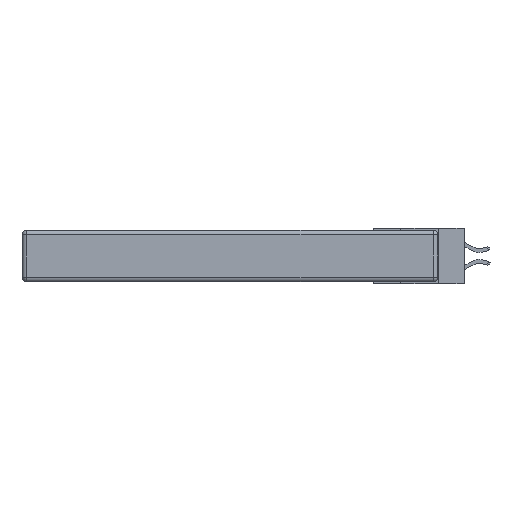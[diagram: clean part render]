
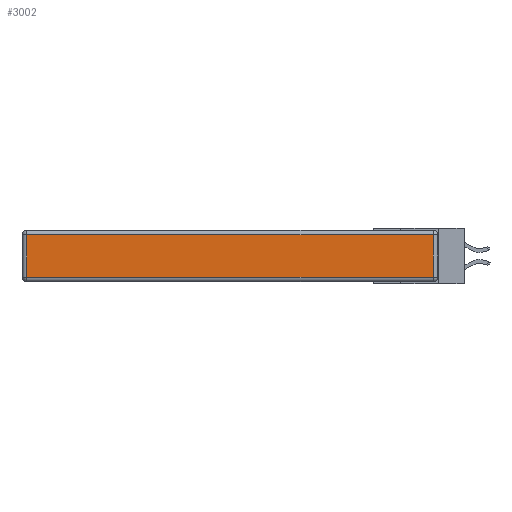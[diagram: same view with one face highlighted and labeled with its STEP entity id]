
A CAD part, left-side view. The second image highlights one B-rep face of the part: STEP entity #3002.
In plain terms, the highlighted planar face has unit normal (-1, 0, 0).
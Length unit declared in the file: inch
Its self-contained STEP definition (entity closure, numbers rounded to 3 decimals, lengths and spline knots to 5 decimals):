
#45 = AXIS2_PLACEMENT_3D ( 'NONE', #1688, #13537, #12020 ) ;
#540 = LINE ( 'NONE', #4034, #991 ) ;
#648 = CARTESIAN_POINT ( 'NONE',  ( 0., 0.03, -0.313 ) ) ;
#930 = ORIENTED_EDGE ( 'NONE', *, *, #17896, .T. ) ;
#991 = VECTOR ( 'NONE', #8322, 39.37008 ) ;
#1546 = ORIENTED_EDGE ( 'NONE', *, *, #5506, .T. ) ;
#1688 = CARTESIAN_POINT ( 'NONE',  ( 0., 0., -0.343 ) ) ;
#3002 = ADVANCED_FACE ( 'NONE', ( #3122 ), #3336, .T. ) ;
#3122 = FACE_OUTER_BOUND ( 'NONE', #18900, .T. ) ;
#3336 = PLANE ( 'NONE',  #45 ) ;
#3992 = CARTESIAN_POINT ( 'NONE',  ( 0., 2.72, -0.343 ) ) ;
#4034 = CARTESIAN_POINT ( 'NONE',  ( 0., 0., -0.313 ) ) ;
#4506 = CARTESIAN_POINT ( 'NONE',  ( 0., 0.03, -0.343 ) ) ;
#5506 = EDGE_CURVE ( 'NONE', #14240, #10334, #11725, .T. ) ;
#6897 = LINE ( 'NONE', #4506, #17632 ) ;
#8322 = DIRECTION ( 'NONE',  ( 0., -1., 0. ) ) ;
#8997 = DIRECTION ( 'NONE',  ( 0., 0., 1. ) ) ;
#9900 = DIRECTION ( 'NONE',  ( 0., 1., 0. ) ) ;
#10334 = VERTEX_POINT ( 'NONE', #18072 ) ;
#10804 = VECTOR ( 'NONE', #11204, 39.37008 ) ;
#11204 = DIRECTION ( 'NONE',  ( 0., 0., -1. ) ) ;
#11336 = VECTOR ( 'NONE', #9900, 39.37008 ) ;
#11417 = ORIENTED_EDGE ( 'NONE', *, *, #14622, .T. ) ;
#11725 = LINE ( 'NONE', #3992, #10804 ) ;
#12020 = DIRECTION ( 'NONE',  ( 0., 0., 1. ) ) ;
#12616 = ORIENTED_EDGE ( 'NONE', *, *, #13039, .T. ) ;
#13039 = EDGE_CURVE ( 'NONE', #18223, #14240, #17281, .T. ) ;
#13537 = DIRECTION ( 'NONE',  ( -1., 0., 0. ) ) ;
#14240 = VERTEX_POINT ( 'NONE', #15225 ) ;
#14622 = EDGE_CURVE ( 'NONE', #10334, #17486, #540, .T. ) ;
#15225 = CARTESIAN_POINT ( 'NONE',  ( 0., 2.72, -0.03 ) ) ;
#17281 = LINE ( 'NONE', #18657, #11336 ) ;
#17381 = CARTESIAN_POINT ( 'NONE',  ( 0., 0.03, -0.03 ) ) ;
#17486 = VERTEX_POINT ( 'NONE', #648 ) ;
#17632 = VECTOR ( 'NONE', #8997, 39.37008 ) ;
#17896 = EDGE_CURVE ( 'NONE', #17486, #18223, #6897, .T. ) ;
#18072 = CARTESIAN_POINT ( 'NONE',  ( 0., 2.72, -0.313 ) ) ;
#18223 = VERTEX_POINT ( 'NONE', #17381 ) ;
#18657 = CARTESIAN_POINT ( 'NONE',  ( 0., 2.75, -0.03 ) ) ;
#18900 = EDGE_LOOP ( 'NONE', ( #11417, #930, #12616, #1546 ) ) ;
